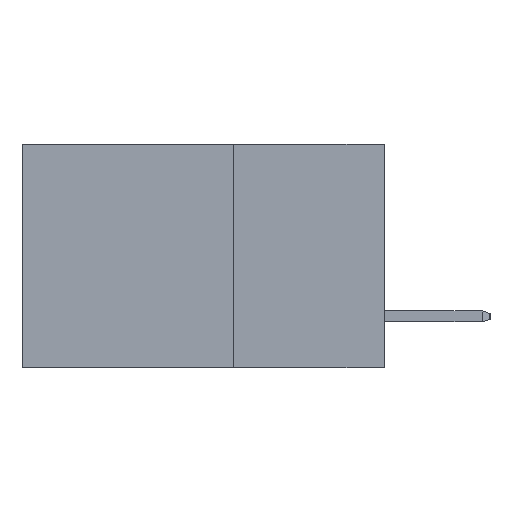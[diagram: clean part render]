
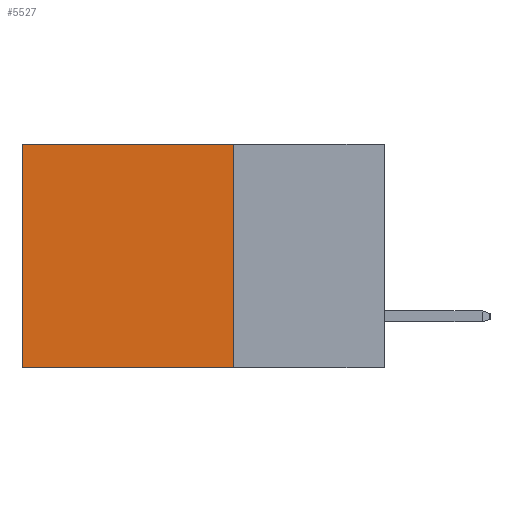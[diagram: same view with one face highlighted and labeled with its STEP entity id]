
A CAD part, left-side view. The second image highlights one B-rep face of the part: STEP entity #5527.
In plain terms, the highlighted planar face has unit normal (-1, 0, 0).
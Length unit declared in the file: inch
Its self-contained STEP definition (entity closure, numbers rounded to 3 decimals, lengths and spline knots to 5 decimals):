
#185 = VECTOR ( 'NONE', #436, 39.37008 ) ;
#436 = DIRECTION ( 'NONE',  ( 0., 1., 0. ) ) ;
#646 = CARTESIAN_POINT ( 'NONE',  ( 0.298, 0.6, 0. ) ) ;
#1098 = CARTESIAN_POINT ( 'NONE',  ( 0.298, 0.6, -0.37 ) ) ;
#1371 = EDGE_CURVE ( 'NONE', #2907, #15111, #4369, .T. ) ;
#1549 = LINE ( 'NONE', #17898, #18151 ) ;
#2210 = DIRECTION ( 'NONE',  ( 0., 0., -1. ) ) ;
#2907 = VERTEX_POINT ( 'NONE', #12737 ) ;
#4160 = ORIENTED_EDGE ( 'NONE', *, *, #9447, .T. ) ;
#4369 = LINE ( 'NONE', #5369, #185 ) ;
#4420 = PLANE ( 'NONE',  #9534 ) ;
#5080 = LINE ( 'NONE', #18352, #16969 ) ;
#5122 = ORIENTED_EDGE ( 'NONE', *, *, #19266, .F. ) ;
#5191 = LINE ( 'NONE', #646, #13424 ) ;
#5271 = EDGE_CURVE ( 'NONE', #18461, #15111, #5191, .T. ) ;
#5369 = CARTESIAN_POINT ( 'NONE',  ( 0.298, 0.25, -0.37 ) ) ;
#5527 = ADVANCED_FACE ( 'NONE', ( #8570 ), #4420, .F. ) ;
#5999 = CARTESIAN_POINT ( 'NONE',  ( 0.298, 0.25, 0. ) ) ;
#6016 = EDGE_LOOP ( 'NONE', ( #19881, #17210, #5122, #4160 ) ) ;
#7476 = DIRECTION ( 'NONE',  ( 0., 1., 0. ) ) ;
#7561 = DIRECTION ( 'NONE',  ( 1., 0., 0. ) ) ;
#8570 = FACE_OUTER_BOUND ( 'NONE', #6016, .T. ) ;
#8580 = DIRECTION ( 'NONE',  ( 0., 0., -1. ) ) ;
#9447 = EDGE_CURVE ( 'NONE', #14038, #18461, #5080, .T. ) ;
#9534 = AXIS2_PLACEMENT_3D ( 'NONE', #5999, #7561, #18436 ) ;
#12323 = CARTESIAN_POINT ( 'NONE',  ( 0.298, 0.25, 0. ) ) ;
#12737 = CARTESIAN_POINT ( 'NONE',  ( 0.298, 0.25, -0.37 ) ) ;
#13424 = VECTOR ( 'NONE', #2210, 39.37008 ) ;
#13594 = CARTESIAN_POINT ( 'NONE',  ( 0.298, 0.6, 0. ) ) ;
#14038 = VERTEX_POINT ( 'NONE', #12323 ) ;
#15111 = VERTEX_POINT ( 'NONE', #1098 ) ;
#16969 = VECTOR ( 'NONE', #7476, 39.37008 ) ;
#17210 = ORIENTED_EDGE ( 'NONE', *, *, #1371, .F. ) ;
#17898 = CARTESIAN_POINT ( 'NONE',  ( 0.298, 0.25, 0. ) ) ;
#18151 = VECTOR ( 'NONE', #8580, 39.37008 ) ;
#18352 = CARTESIAN_POINT ( 'NONE',  ( 0.298, 0.25, 0. ) ) ;
#18436 = DIRECTION ( 'NONE',  ( 0., 0., -1. ) ) ;
#18461 = VERTEX_POINT ( 'NONE', #13594 ) ;
#19266 = EDGE_CURVE ( 'NONE', #14038, #2907, #1549, .T. ) ;
#19881 = ORIENTED_EDGE ( 'NONE', *, *, #5271, .T. ) ;
